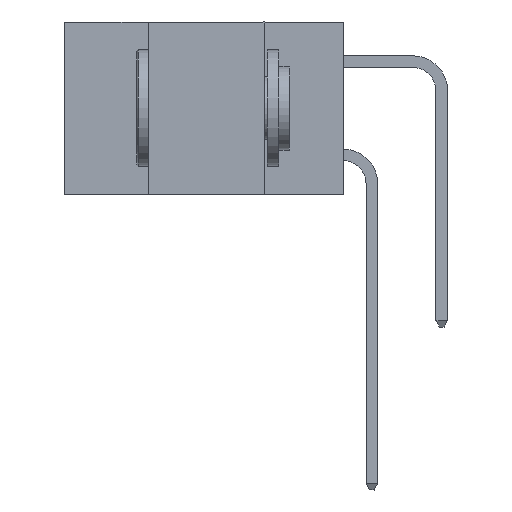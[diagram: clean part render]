
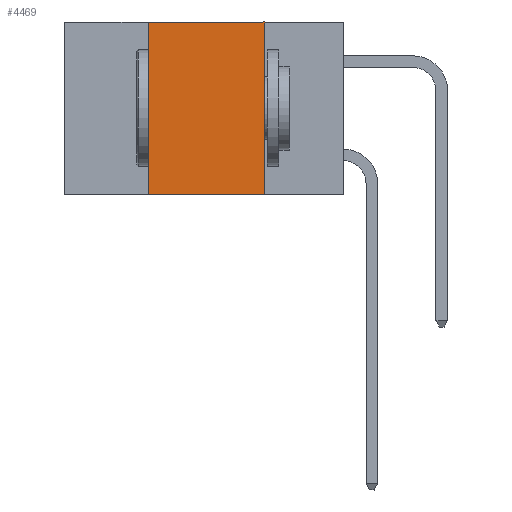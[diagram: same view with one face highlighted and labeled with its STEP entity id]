
A CAD part, left-side view. The second image highlights one B-rep face of the part: STEP entity #4469.
In plain terms, the highlighted planar face has unit normal (-1, 0, 0).
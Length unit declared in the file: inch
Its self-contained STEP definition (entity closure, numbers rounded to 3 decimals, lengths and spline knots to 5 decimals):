
#208 = DIRECTION ( 'NONE',  ( 0., -1., 0. ) ) ;
#681 = VECTOR ( 'NONE', #7537, 39.37008 ) ;
#1116 = LINE ( 'NONE', #7458, #8068 ) ;
#1318 = EDGE_CURVE ( 'NONE', #12045, #10166, #3299, .T. ) ;
#1559 = DIRECTION ( 'NONE',  ( 1., 0., 0. ) ) ;
#1776 = CARTESIAN_POINT ( 'NONE',  ( 0., 0.17, 0. ) ) ;
#1850 = EDGE_CURVE ( 'NONE', #5481, #10166, #1116, .T. ) ;
#2438 = CARTESIAN_POINT ( 'NONE',  ( 0., 0.17, -0.37 ) ) ;
#2686 = CARTESIAN_POINT ( 'NONE',  ( 0., 0.6, 0. ) ) ;
#2891 = VECTOR ( 'NONE', #6004, 39.37008 ) ;
#3299 = LINE ( 'NONE', #4496, #681 ) ;
#3585 = ORIENTED_EDGE ( 'NONE', *, *, #12825, .F. ) ;
#3844 = CARTESIAN_POINT ( 'NONE',  ( 0., 0.42, -0.37 ) ) ;
#4469 = ADVANCED_FACE ( 'NONE', ( #8958 ), #13131, .F. ) ;
#4496 = CARTESIAN_POINT ( 'NONE',  ( 0., 0.17, -0.37 ) ) ;
#5381 = AXIS2_PLACEMENT_3D ( 'NONE', #2686, #1559, #9021 ) ;
#5481 = VERTEX_POINT ( 'NONE', #3844 ) ;
#6004 = DIRECTION ( 'NONE',  ( 0., -1., 0. ) ) ;
#6304 = EDGE_LOOP ( 'NONE', ( #11953, #10537, #3585, #12466 ) ) ;
#7458 = CARTESIAN_POINT ( 'NONE',  ( 0., 0.6, -0.37 ) ) ;
#7537 = DIRECTION ( 'NONE',  ( 0., 0., -1. ) ) ;
#8068 = VECTOR ( 'NONE', #208, 39.37008 ) ;
#8958 = FACE_OUTER_BOUND ( 'NONE', #6304, .T. ) ;
#9021 = DIRECTION ( 'NONE',  ( 0., 0., -1. ) ) ;
#9026 = DIRECTION ( 'NONE',  ( 0., 0., 1. ) ) ;
#9131 = CARTESIAN_POINT ( 'NONE',  ( 0., 0.6, 0. ) ) ;
#9282 = VERTEX_POINT ( 'NONE', #12097 ) ;
#9792 = VECTOR ( 'NONE', #9026, 39.37008 ) ;
#10166 = VERTEX_POINT ( 'NONE', #2438 ) ;
#10191 = LINE ( 'NONE', #12300, #9792 ) ;
#10537 = ORIENTED_EDGE ( 'NONE', *, *, #11181, .F. ) ;
#11181 = EDGE_CURVE ( 'NONE', #9282, #12045, #13571, .T. ) ;
#11953 = ORIENTED_EDGE ( 'NONE', *, *, #1318, .F. ) ;
#12045 = VERTEX_POINT ( 'NONE', #1776 ) ;
#12097 = CARTESIAN_POINT ( 'NONE',  ( 0., 0.42, 0. ) ) ;
#12300 = CARTESIAN_POINT ( 'NONE',  ( 0., 0.42, -0.37 ) ) ;
#12466 = ORIENTED_EDGE ( 'NONE', *, *, #1850, .T. ) ;
#12825 = EDGE_CURVE ( 'NONE', #5481, #9282, #10191, .T. ) ;
#13131 = PLANE ( 'NONE',  #5381 ) ;
#13571 = LINE ( 'NONE', #9131, #2891 ) ;
